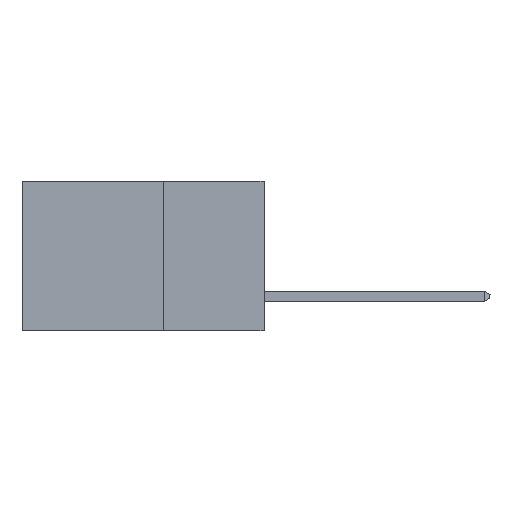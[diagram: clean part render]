
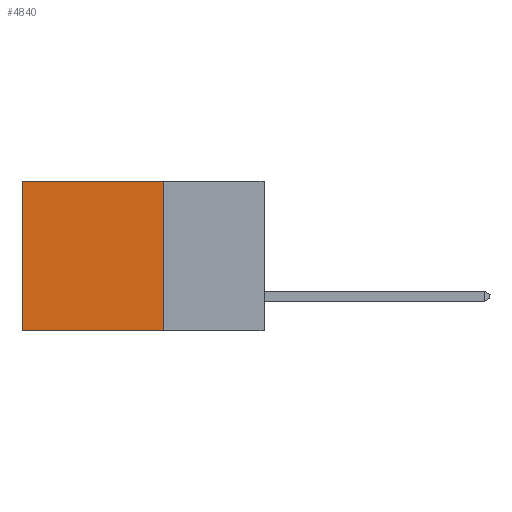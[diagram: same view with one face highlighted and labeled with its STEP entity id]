
A CAD part, left-side view. The second image highlights one B-rep face of the part: STEP entity #4840.
In plain terms, the highlighted planar face has unit normal (-1, 0, 0).
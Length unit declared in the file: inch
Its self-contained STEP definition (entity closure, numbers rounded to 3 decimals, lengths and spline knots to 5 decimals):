
#134 = VECTOR ( 'NONE', #11375, 39.37008 ) ;
#751 = EDGE_CURVE ( 'NONE', #5121, #10609, #1855, .T. ) ;
#769 = ORIENTED_EDGE ( 'NONE', *, *, #11718, .F. ) ;
#1198 = LINE ( 'NONE', #9761, #4757 ) ;
#1404 = ORIENTED_EDGE ( 'NONE', *, *, #4293, .T. ) ;
#1496 = CARTESIAN_POINT ( 'NONE',  ( 0.2615, 0.6, -0.37 ) ) ;
#1855 = LINE ( 'NONE', #4951, #3315 ) ;
#2233 = VERTEX_POINT ( 'NONE', #4551 ) ;
#2731 = VECTOR ( 'NONE', #6598, 39.37008 ) ;
#3285 = CARTESIAN_POINT ( 'NONE',  ( 0.2615, 0.6, -0.37 ) ) ;
#3315 = VECTOR ( 'NONE', #11566, 39.37008 ) ;
#3628 = CARTESIAN_POINT ( 'NONE',  ( 0.2615, 0.25, -0.37 ) ) ;
#3651 = EDGE_CURVE ( 'NONE', #2233, #9112, #1198, .T. ) ;
#4293 = EDGE_CURVE ( 'NONE', #9112, #10609, #7622, .T. ) ;
#4551 = CARTESIAN_POINT ( 'NONE',  ( 0.2615, 0.25, 0. ) ) ;
#4757 = VECTOR ( 'NONE', #10791, 39.37008 ) ;
#4840 = ADVANCED_FACE ( 'NONE', ( #7478 ), #6526, .F. ) ;
#4951 = CARTESIAN_POINT ( 'NONE',  ( 0.2615, 0.25, -0.37 ) ) ;
#5121 = VERTEX_POINT ( 'NONE', #9240 ) ;
#5692 = ORIENTED_EDGE ( 'NONE', *, *, #751, .F. ) ;
#5982 = DIRECTION ( 'NONE',  ( 0., 0., -1. ) ) ;
#6526 = PLANE ( 'NONE',  #8710 ) ;
#6598 = DIRECTION ( 'NONE',  ( 0., 0., -1. ) ) ;
#7453 = LINE ( 'NONE', #10203, #134 ) ;
#7478 = FACE_OUTER_BOUND ( 'NONE', #10554, .T. ) ;
#7622 = LINE ( 'NONE', #1496, #2731 ) ;
#8500 = ORIENTED_EDGE ( 'NONE', *, *, #3651, .T. ) ;
#8622 = CARTESIAN_POINT ( 'NONE',  ( 0.2615, 0.6, 0. ) ) ;
#8710 = AXIS2_PLACEMENT_3D ( 'NONE', #3628, #12535, #5982 ) ;
#9112 = VERTEX_POINT ( 'NONE', #8622 ) ;
#9240 = CARTESIAN_POINT ( 'NONE',  ( 0.2615, 0.25, -0.37 ) ) ;
#9761 = CARTESIAN_POINT ( 'NONE',  ( 0.2615, 0.25, 0. ) ) ;
#10203 = CARTESIAN_POINT ( 'NONE',  ( 0.2615, 0.25, -0.37 ) ) ;
#10554 = EDGE_LOOP ( 'NONE', ( #1404, #5692, #769, #8500 ) ) ;
#10609 = VERTEX_POINT ( 'NONE', #3285 ) ;
#10791 = DIRECTION ( 'NONE',  ( 0., 1., 0. ) ) ;
#11375 = DIRECTION ( 'NONE',  ( 0., 0., -1. ) ) ;
#11566 = DIRECTION ( 'NONE',  ( 0., 1., 0. ) ) ;
#11718 = EDGE_CURVE ( 'NONE', #2233, #5121, #7453, .T. ) ;
#12535 = DIRECTION ( 'NONE',  ( 1., 0., 0. ) ) ;
